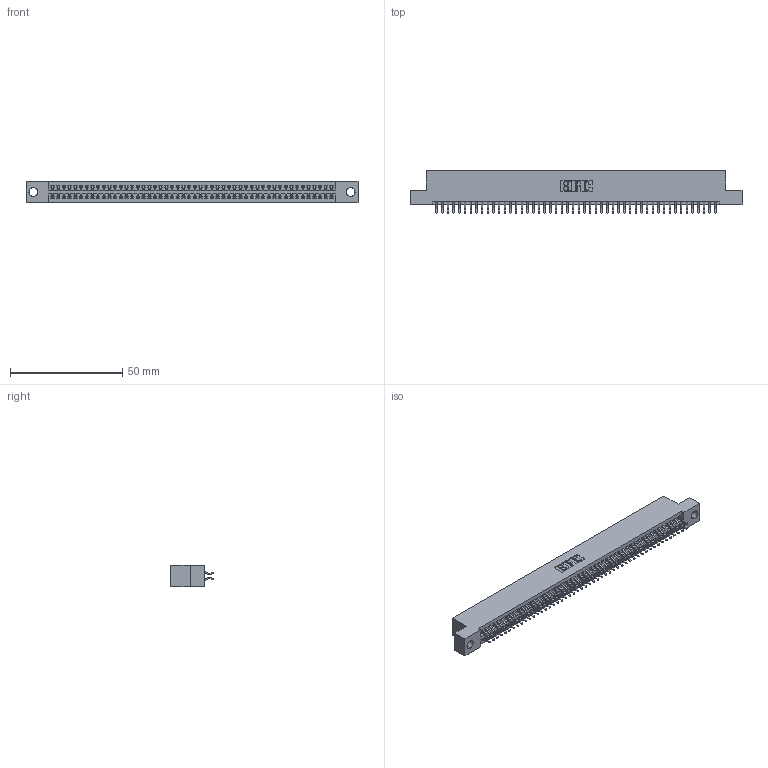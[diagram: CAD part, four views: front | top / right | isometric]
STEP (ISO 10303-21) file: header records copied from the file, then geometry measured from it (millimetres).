
FILE_DESCRIPTION (( 'STEP AP203' ), '1' );
FILE_NAME ('345-100-556-204.STEP', '2021-05-20T19:03:08', ( '' ), ( '' ), 'SwSTEP 2.0', 'SolidWorks 2020', '' );
FILE_SCHEMA (( 'CONFIG_CONTROL_DESIGN' ));
Length unit declared in the file: inch
Products named in the file (3): 345-100-556-204; 345 Part_Flush Mounting Lugs - 0.156 Dia-TI; 345-292-001_556 Tail
Assembly tree (101 placements, depth 2):
  345-100-556-204
    345 Part_Flush Mounting Lugs - 0.156 Dia-TI
    345-292-001_556 Tail  x100
Bounding box: 148.21 x 19.24 x 9.4 mm (x, y, z)
Volume: 14361.5 mm3; surface area: 21147.7 mm2
Topology: 101 solids, 101 shells, 5740 faces, 17077 edges, 11250 vertices
Faces by surface type: plane 3794, cylinder 1946
Entity records: 38793 total; most frequent: CARTESIAN_POINT 6514, ORIENTED_EDGE 6434, DIRECTION 5721, EDGE_CURVE 3217, LINE 2877, VECTOR 2877, VERTEX_POINT 2142, AXIS2_PLACEMENT_3D 1422
